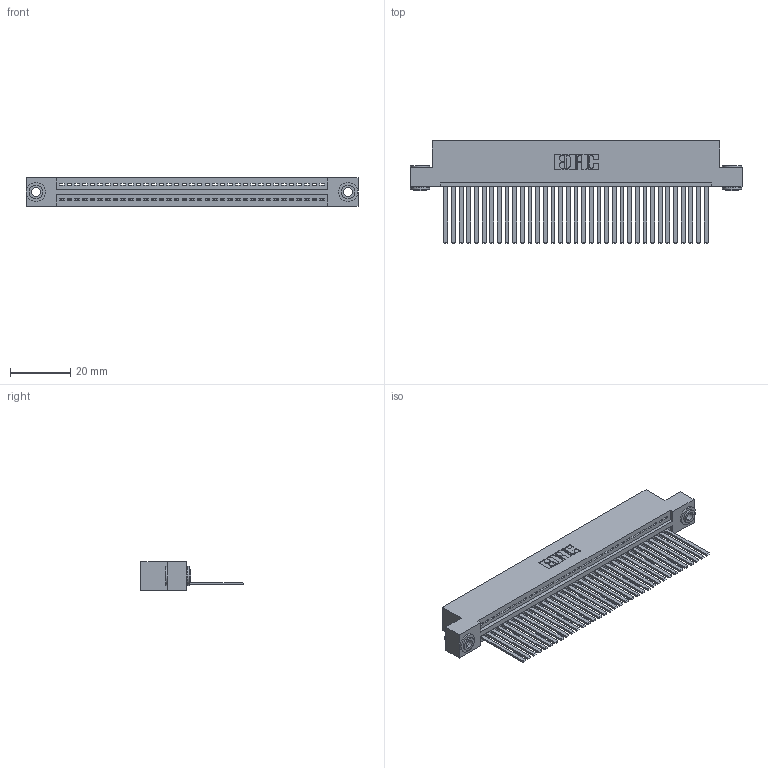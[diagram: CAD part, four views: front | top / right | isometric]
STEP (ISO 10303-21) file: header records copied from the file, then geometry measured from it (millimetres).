
FILE_DESCRIPTION (( 'STEP AP203' ), '1' );
FILE_NAME ('395-035-544-103.STEP', '2019-10-19T19:59:07', ( '' ), ( '' ), 'SwSTEP 2.0', 'SolidWorks 2016', '' );
FILE_SCHEMA (( 'CONFIG_CONTROL_DESIGN' ));
Length unit declared in the file: inch
Products named in the file (4): 395-035-544-103; 345-250-002_345-250-002-102; 345 Part_Flush Mounting Lugs - 0.156 Dia-TH; 345-292-001_345-293-144
Assembly tree (38 placements, depth 2):
  395-035-544-103
    345 Part_Flush Mounting Lugs - 0.156 Dia-TH
    345-292-001_345-293-144  x35
    345-250-002_345-250-002-102  x2
Bounding box: 110.11 x 33.96 x 9.4 mm (x, y, z)
Volume: 10825.7 mm3; surface area: 15722.6 mm2
Topology: 38 solids, 38 shells, 1984 faces, 5947 edges, 3914 vertices
Faces by surface type: plane 1350, cylinder 626, cone 8
Entity records: 27750 total; most frequent: CARTESIAN_POINT 4784, ORIENTED_EDGE 4746, DIRECTION 4217, EDGE_CURVE 2373, VECTOR 2081, LINE 2081, VERTEX_POINT 1578, AXIS2_PLACEMENT_3D 1068
